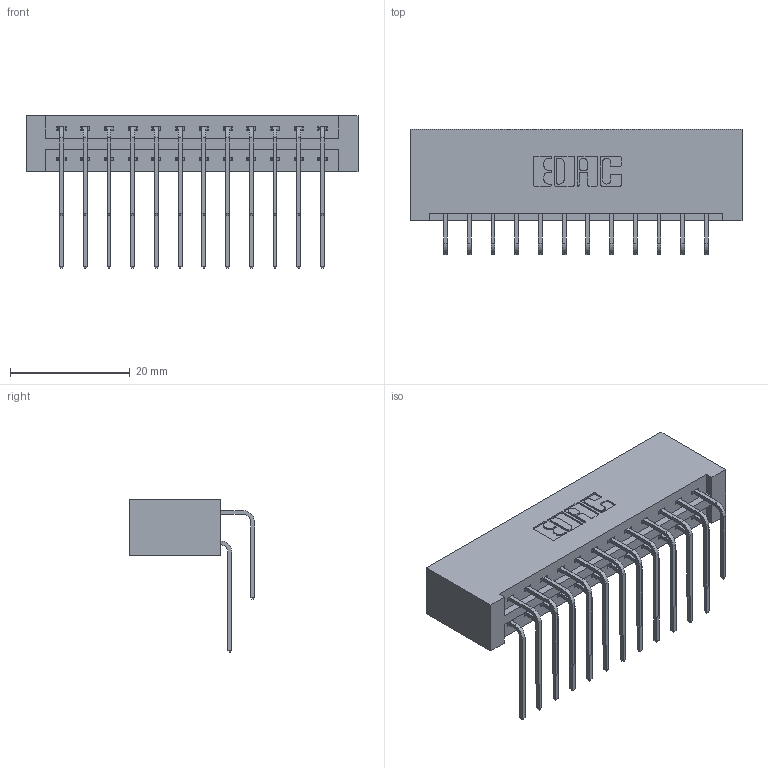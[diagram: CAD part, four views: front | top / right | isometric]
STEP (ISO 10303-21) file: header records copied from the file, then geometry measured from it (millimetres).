
FILE_DESCRIPTION (( 'STEP AP203' ), '1' );
FILE_NAME ('387-024-559-201.STEP', '2019-10-16T19:04:43', ( '' ), ( '' ), 'SwSTEP 2.0', 'SolidWorks 2016', '' );
FILE_SCHEMA (( 'CONFIG_CONTROL_DESIGN' ));
Length unit declared in the file: inch
Products named in the file (4): 337 Part_No Mounting Lugs; 387-024-559-201; 345-292-001_558 559 Tail - 1; 345-292-001_559 Tail - 2
Assembly tree (25 placements, depth 2):
  387-024-559-201
    337 Part_No Mounting Lugs
    345-292-001_558 559 Tail - 1  x12
    345-292-001_559 Tail - 2  x12
Bounding box: 55.42 x 20.9 x 25.53 mm (x, y, z)
Volume: 6340.8 mm3; surface area: 7628.1 mm2
Topology: 25 solids, 25 shells, 1450 faces, 4295 edges, 2830 vertices
Faces by surface type: plane 1026, cylinder 424
Entity records: 14691 total; most frequent: CARTESIAN_POINT 2545, ORIENTED_EDGE 2430, DIRECTION 2195, EDGE_CURVE 1215, LINE 1055, VECTOR 1055, VERTEX_POINT 806, AXIS2_PLACEMENT_3D 570
